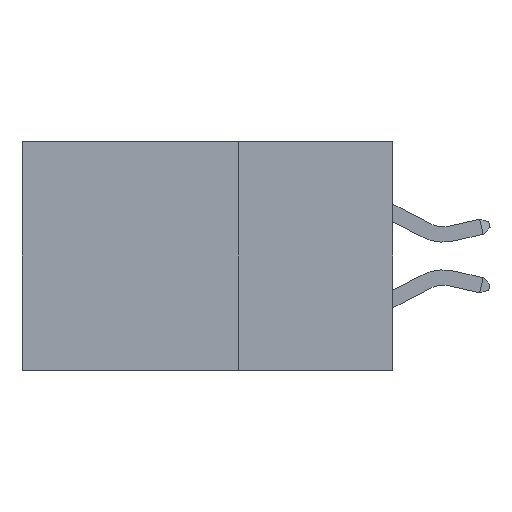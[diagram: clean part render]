
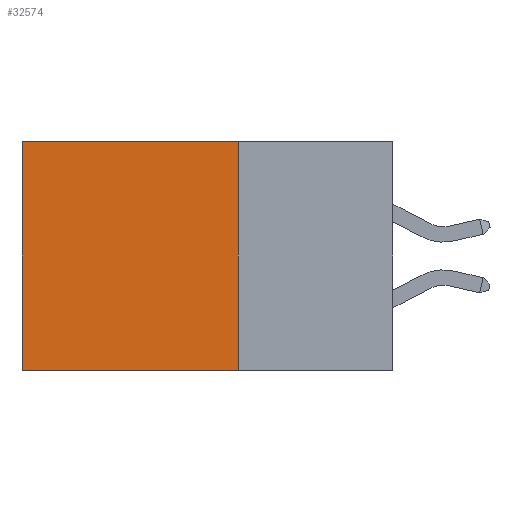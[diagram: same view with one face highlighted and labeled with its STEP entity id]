
A CAD part, left-side view. The second image highlights one B-rep face of the part: STEP entity #32574.
In plain terms, the highlighted planar face has unit normal (-1, 0, 0).
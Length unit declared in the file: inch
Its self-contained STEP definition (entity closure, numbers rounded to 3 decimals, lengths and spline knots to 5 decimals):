
#10 = DIRECTION ( 'NONE',  ( 0., 0., -1. ) ) ;
#505 = VECTOR ( 'NONE', #13492, 39.37008 ) ;
#5404 = EDGE_LOOP ( 'NONE', ( #5867, #30718, #20991, #38517 ) ) ;
#5867 = ORIENTED_EDGE ( 'NONE', *, *, #19278, .T. ) ;
#8881 = CARTESIAN_POINT ( 'NONE',  ( 0.2875, 0.25, 0. ) ) ;
#10144 = DIRECTION ( 'NONE',  ( 0., 1., 0. ) ) ;
#12012 = PLANE ( 'NONE',  #16480 ) ;
#13492 = DIRECTION ( 'NONE',  ( 0., 0., -1. ) ) ;
#14168 = LINE ( 'NONE', #26146, #35618 ) ;
#16062 = CARTESIAN_POINT ( 'NONE',  ( 0.2875, 0.6, 0. ) ) ;
#16445 = LINE ( 'NONE', #16062, #505 ) ;
#16480 = AXIS2_PLACEMENT_3D ( 'NONE', #8881, #23412, #35612 ) ;
#16932 = CARTESIAN_POINT ( 'NONE',  ( 0.2875, 0.25, 0. ) ) ;
#17464 = LINE ( 'NONE', #38682, #17618 ) ;
#17618 = VECTOR ( 'NONE', #26511, 39.37008 ) ;
#19278 = EDGE_CURVE ( 'NONE', #22094, #31994, #16445, .T. ) ;
#20292 = EDGE_CURVE ( 'NONE', #37838, #25641, #14168, .T. ) ;
#20608 = VECTOR ( 'NONE', #10144, 39.37008 ) ;
#20991 = ORIENTED_EDGE ( 'NONE', *, *, #20292, .F. ) ;
#22094 = VERTEX_POINT ( 'NONE', #31854 ) ;
#22523 = CARTESIAN_POINT ( 'NONE',  ( 0.2875, 0.25, -0.37 ) ) ;
#23412 = DIRECTION ( 'NONE',  ( 1., 0., 0. ) ) ;
#25641 = VERTEX_POINT ( 'NONE', #22523 ) ;
#26146 = CARTESIAN_POINT ( 'NONE',  ( 0.2875, 0.25, 0. ) ) ;
#26511 = DIRECTION ( 'NONE',  ( 0., 1., 0. ) ) ;
#27817 = EDGE_CURVE ( 'NONE', #37838, #22094, #27832, .T. ) ;
#27832 = LINE ( 'NONE', #37051, #20608 ) ;
#29320 = FACE_OUTER_BOUND ( 'NONE', #5404, .T. ) ;
#30168 = EDGE_CURVE ( 'NONE', #25641, #31994, #17464, .T. ) ;
#30718 = ORIENTED_EDGE ( 'NONE', *, *, #30168, .F. ) ;
#31854 = CARTESIAN_POINT ( 'NONE',  ( 0.2875, 0.6, 0. ) ) ;
#31994 = VERTEX_POINT ( 'NONE', #37248 ) ;
#32574 = ADVANCED_FACE ( 'NONE', ( #29320 ), #12012, .F. ) ;
#35612 = DIRECTION ( 'NONE',  ( 0., 0., -1. ) ) ;
#35618 = VECTOR ( 'NONE', #10, 39.37008 ) ;
#37051 = CARTESIAN_POINT ( 'NONE',  ( 0.2875, 0.25, 0. ) ) ;
#37248 = CARTESIAN_POINT ( 'NONE',  ( 0.2875, 0.6, -0.37 ) ) ;
#37838 = VERTEX_POINT ( 'NONE', #16932 ) ;
#38517 = ORIENTED_EDGE ( 'NONE', *, *, #27817, .T. ) ;
#38682 = CARTESIAN_POINT ( 'NONE',  ( 0.2875, 0.25, -0.37 ) ) ;
